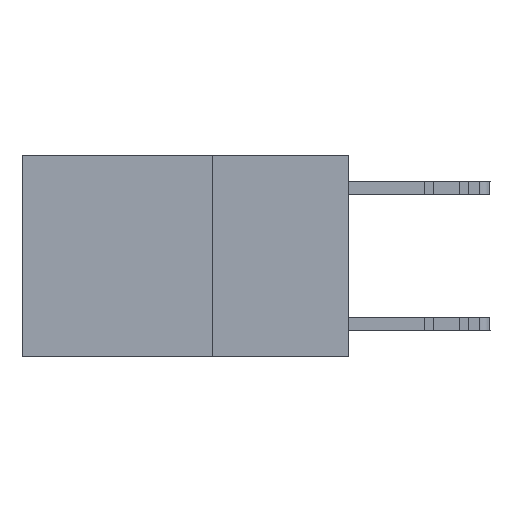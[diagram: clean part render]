
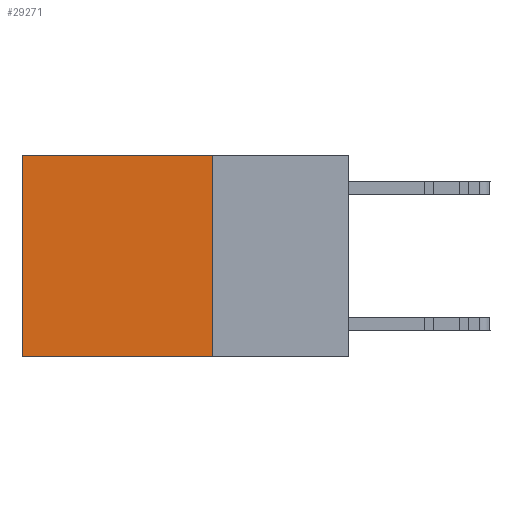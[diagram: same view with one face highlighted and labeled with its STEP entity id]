
A CAD part, left-side view. The second image highlights one B-rep face of the part: STEP entity #29271.
In plain terms, the highlighted planar face has unit normal (-1, 0, 0).
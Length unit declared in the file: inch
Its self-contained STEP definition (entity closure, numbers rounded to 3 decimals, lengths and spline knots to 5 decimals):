
#1352 = CARTESIAN_POINT ( 'NONE',  ( 0.2625, 0.25, -0.37 ) ) ;
#3709 = AXIS2_PLACEMENT_3D ( 'NONE', #25754, #30922, #4390 ) ;
#4174 = CARTESIAN_POINT ( 'NONE',  ( 0.2625, 0.25, 0. ) ) ;
#4390 = DIRECTION ( 'NONE',  ( 0., 0., -1. ) ) ;
#5613 = CARTESIAN_POINT ( 'NONE',  ( 0.2625, 0.25, 0. ) ) ;
#6660 = VECTOR ( 'NONE', #7640, 39.37008 ) ;
#7119 = DIRECTION ( 'NONE',  ( 0., 1., 0. ) ) ;
#7161 = CARTESIAN_POINT ( 'NONE',  ( 0.2625, 0.6, 0. ) ) ;
#7179 = VECTOR ( 'NONE', #8144, 39.37008 ) ;
#7542 = VECTOR ( 'NONE', #13458, 39.37008 ) ;
#7640 = DIRECTION ( 'NONE',  ( 0., 0., -1. ) ) ;
#8144 = DIRECTION ( 'NONE',  ( 0., 0., -1. ) ) ;
#9806 = VERTEX_POINT ( 'NONE', #24796 ) ;
#10902 = CARTESIAN_POINT ( 'NONE',  ( 0.2625, 0.6, 0. ) ) ;
#11149 = VECTOR ( 'NONE', #7119, 39.37008 ) ;
#12079 = EDGE_CURVE ( 'NONE', #15336, #18732, #19070, .T. ) ;
#12859 = LINE ( 'NONE', #5613, #7179 ) ;
#13284 = ORIENTED_EDGE ( 'NONE', *, *, #21728, .F. ) ;
#13458 = DIRECTION ( 'NONE',  ( 0., 1., 0. ) ) ;
#14727 = ORIENTED_EDGE ( 'NONE', *, *, #28133, .F. ) ;
#15336 = VERTEX_POINT ( 'NONE', #4174 ) ;
#16599 = LINE ( 'NONE', #7161, #6660 ) ;
#18732 = VERTEX_POINT ( 'NONE', #10902 ) ;
#19070 = LINE ( 'NONE', #28644, #11149 ) ;
#19199 = VERTEX_POINT ( 'NONE', #25601 ) ;
#21728 = EDGE_CURVE ( 'NONE', #19199, #9806, #29474, .T. ) ;
#21916 = ORIENTED_EDGE ( 'NONE', *, *, #12079, .T. ) ;
#23413 = PLANE ( 'NONE',  #3709 ) ;
#24025 = FACE_OUTER_BOUND ( 'NONE', #24920, .T. ) ;
#24796 = CARTESIAN_POINT ( 'NONE',  ( 0.2625, 0.6, -0.37 ) ) ;
#24920 = EDGE_LOOP ( 'NONE', ( #28688, #13284, #14727, #21916 ) ) ;
#25601 = CARTESIAN_POINT ( 'NONE',  ( 0.2625, 0.25, -0.37 ) ) ;
#25754 = CARTESIAN_POINT ( 'NONE',  ( 0.2625, 0.25, 0. ) ) ;
#28133 = EDGE_CURVE ( 'NONE', #15336, #19199, #12859, .T. ) ;
#28644 = CARTESIAN_POINT ( 'NONE',  ( 0.2625, 0.25, 0. ) ) ;
#28688 = ORIENTED_EDGE ( 'NONE', *, *, #29771, .T. ) ;
#29271 = ADVANCED_FACE ( 'NONE', ( #24025 ), #23413, .F. ) ;
#29474 = LINE ( 'NONE', #1352, #7542 ) ;
#29771 = EDGE_CURVE ( 'NONE', #18732, #9806, #16599, .T. ) ;
#30922 = DIRECTION ( 'NONE',  ( 1., 0., 0. ) ) ;
